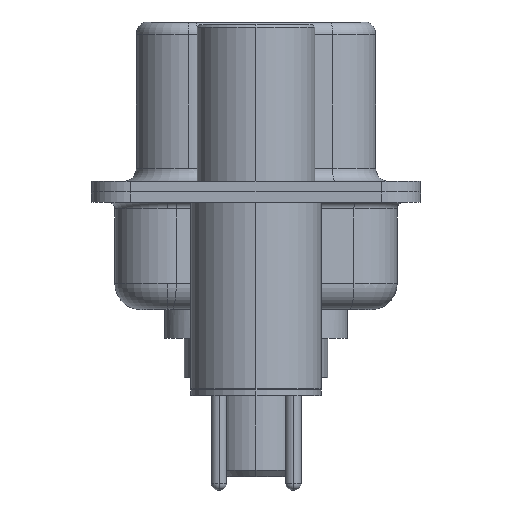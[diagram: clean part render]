
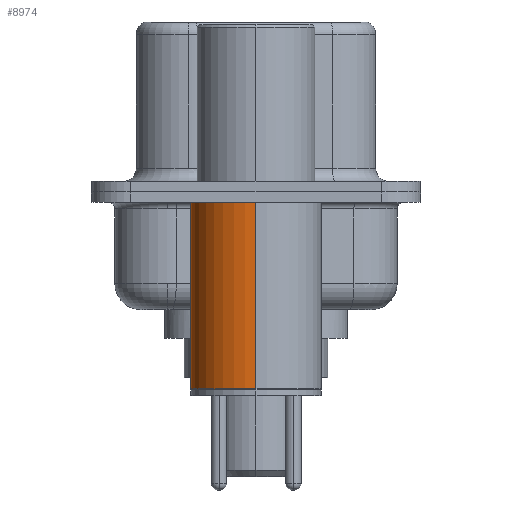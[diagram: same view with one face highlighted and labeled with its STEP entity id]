
A CAD part, left-side view. The second image highlights one B-rep face of the part: STEP entity #8974.
In plain terms, the highlighted cylindrical face has radius 2.5 mm (diameter 5 mm), a partial arc.
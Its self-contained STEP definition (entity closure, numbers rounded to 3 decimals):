
#204 = ORIENTED_EDGE ( 'NONE', *, *, #2303, .F. ) ;
#510 = CARTESIAN_POINT ( 'NONE',  ( 0., 0., -0.4 ) ) ;
#559 = ORIENTED_EDGE ( 'NONE', *, *, #2156, .T. ) ;
#1327 = CARTESIAN_POINT ( 'NONE',  ( 2.5, 0., -7.525 ) ) ;
#2129 = VERTEX_POINT ( 'NONE', #12570 ) ;
#2156 = EDGE_CURVE ( 'NONE', #2281, #5694, #9442, .T. ) ;
#2206 = EDGE_CURVE ( 'NONE', #5694, #13425, #8281, .T. ) ;
#2279 = EDGE_CURVE ( 'NONE', #2129, #13425, #14357, .T. ) ;
#2281 = VERTEX_POINT ( 'NONE', #1327 ) ;
#2303 = EDGE_CURVE ( 'NONE', #2281, #2129, #7507, .T. ) ;
#2348 = DIRECTION ( 'NONE',  ( 1., 0., 0. ) ) ;
#3001 = CYLINDRICAL_SURFACE ( 'NONE', #11248, 2.5 ) ;
#3732 = AXIS2_PLACEMENT_3D ( 'NONE', #8129, #10684, #5468 ) ;
#3947 = ORIENTED_EDGE ( 'NONE', *, *, #2279, .F. ) ;
#4642 = DIRECTION ( 'NONE',  ( 0., 0., 1. ) ) ;
#4971 = CARTESIAN_POINT ( 'NONE',  ( 2.5, 0., 0.581 ) ) ;
#5072 = DIRECTION ( 'NONE',  ( 1., 0., 0. ) ) ;
#5080 = DIRECTION ( 'NONE',  ( 0., 0., 1. ) ) ;
#5468 = DIRECTION ( 'NONE',  ( 1., 0., 0. ) ) ;
#5694 = VERTEX_POINT ( 'NONE', #12453 ) ;
#6579 = CARTESIAN_POINT ( 'NONE',  ( -2.5, 0., 0.581 ) ) ;
#7106 = VECTOR ( 'NONE', #5080, 1000. ) ;
#7507 = LINE ( 'NONE', #4971, #7106 ) ;
#8129 = CARTESIAN_POINT ( 'NONE',  ( 0., 0., -7.525 ) ) ;
#8281 = LINE ( 'NONE', #6579, #11552 ) ;
#8974 = ADVANCED_FACE ( 'NONE', ( #9617 ), #3001, .T. ) ;
#9442 = CIRCLE ( 'NONE', #3732, 2.5 ) ;
#9617 = FACE_OUTER_BOUND ( 'NONE', #10896, .T. ) ;
#10684 = DIRECTION ( 'NONE',  ( 0., 0., 1. ) ) ;
#10896 = EDGE_LOOP ( 'NONE', ( #559, #15129, #3947, #204 ) ) ;
#10912 = CARTESIAN_POINT ( 'NONE',  ( -2.5, 0., -0.4 ) ) ;
#11248 = AXIS2_PLACEMENT_3D ( 'NONE', #14973, #11323, #5072 ) ;
#11323 = DIRECTION ( 'NONE',  ( 0., 0., 1. ) ) ;
#11552 = VECTOR ( 'NONE', #4642, 1000. ) ;
#12050 = AXIS2_PLACEMENT_3D ( 'NONE', #510, #14546, #2348 ) ;
#12453 = CARTESIAN_POINT ( 'NONE',  ( -2.5, 0., -7.525 ) ) ;
#12570 = CARTESIAN_POINT ( 'NONE',  ( 2.5, 0., -0.4 ) ) ;
#13425 = VERTEX_POINT ( 'NONE', #10912 ) ;
#14357 = CIRCLE ( 'NONE', #12050, 2.5 ) ;
#14546 = DIRECTION ( 'NONE',  ( 0., 0., 1. ) ) ;
#14973 = CARTESIAN_POINT ( 'NONE',  ( 0., 0., 0.581 ) ) ;
#15129 = ORIENTED_EDGE ( 'NONE', *, *, #2206, .T. ) ;
